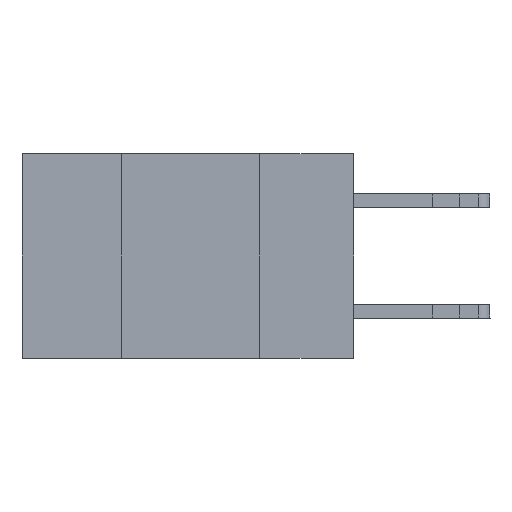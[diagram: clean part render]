
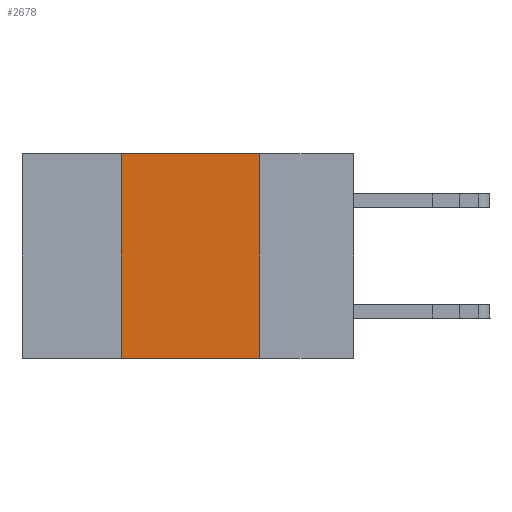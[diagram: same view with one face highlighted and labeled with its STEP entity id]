
A CAD part, left-side view. The second image highlights one B-rep face of the part: STEP entity #2678.
In plain terms, the highlighted planar face has unit normal (-1, 0, 0).
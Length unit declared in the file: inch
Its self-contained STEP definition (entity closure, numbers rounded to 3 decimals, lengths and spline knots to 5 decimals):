
#125 = CARTESIAN_POINT ( 'NONE',  ( 0., 0.6, -0.37 ) ) ;
#500 = FACE_OUTER_BOUND ( 'NONE', #3362, .T. ) ;
#575 = PLANE ( 'NONE',  #9964 ) ;
#965 = LINE ( 'NONE', #12257, #12433 ) ;
#1796 = ORIENTED_EDGE ( 'NONE', *, *, #3652, .F. ) ;
#2283 = VECTOR ( 'NONE', #12940, 39.37008 ) ;
#2678 = ADVANCED_FACE ( 'NONE', ( #500 ), #575, .F. ) ;
#3362 = EDGE_LOOP ( 'NONE', ( #1796, #6665, #6150, #10160 ) ) ;
#3477 = CARTESIAN_POINT ( 'NONE',  ( 0., 0.42, -0.37 ) ) ;
#3588 = VECTOR ( 'NONE', #4647, 39.37008 ) ;
#3652 = EDGE_CURVE ( 'NONE', #11167, #9897, #965, .T. ) ;
#4084 = CARTESIAN_POINT ( 'NONE',  ( 0., 0.17, -0.37 ) ) ;
#4290 = DIRECTION ( 'NONE',  ( 0., 0., -1. ) ) ;
#4377 = CARTESIAN_POINT ( 'NONE',  ( 0., 0.42, 0. ) ) ;
#4647 = DIRECTION ( 'NONE',  ( 0., -1., 0. ) ) ;
#5505 = VERTEX_POINT ( 'NONE', #3477 ) ;
#5913 = CARTESIAN_POINT ( 'NONE',  ( 0., 0.17, 0. ) ) ;
#6150 = ORIENTED_EDGE ( 'NONE', *, *, #13628, .F. ) ;
#6251 = VECTOR ( 'NONE', #9463, 39.37008 ) ;
#6665 = ORIENTED_EDGE ( 'NONE', *, *, #8636, .F. ) ;
#8440 = VERTEX_POINT ( 'NONE', #14270 ) ;
#8636 = EDGE_CURVE ( 'NONE', #8440, #11167, #16098, .T. ) ;
#8903 = LINE ( 'NONE', #125, #2283 ) ;
#9463 = DIRECTION ( 'NONE',  ( 0., 0., 1. ) ) ;
#9625 = LINE ( 'NONE', #4377, #6251 ) ;
#9731 = DIRECTION ( 'NONE',  ( 0., 0., -1. ) ) ;
#9897 = VERTEX_POINT ( 'NONE', #4084 ) ;
#9964 = AXIS2_PLACEMENT_3D ( 'NONE', #10852, #15750, #4290 ) ;
#10160 = ORIENTED_EDGE ( 'NONE', *, *, #14320, .T. ) ;
#10852 = CARTESIAN_POINT ( 'NONE',  ( 0., 0.6, 0. ) ) ;
#11167 = VERTEX_POINT ( 'NONE', #5913 ) ;
#12257 = CARTESIAN_POINT ( 'NONE',  ( 0., 0.17, 0. ) ) ;
#12433 = VECTOR ( 'NONE', #9731, 39.37008 ) ;
#12940 = DIRECTION ( 'NONE',  ( 0., -1., 0. ) ) ;
#13628 = EDGE_CURVE ( 'NONE', #5505, #8440, #9625, .T. ) ;
#14270 = CARTESIAN_POINT ( 'NONE',  ( 0., 0.42, 0. ) ) ;
#14320 = EDGE_CURVE ( 'NONE', #5505, #9897, #8903, .T. ) ;
#14856 = CARTESIAN_POINT ( 'NONE',  ( 0., 0.6, 0. ) ) ;
#15750 = DIRECTION ( 'NONE',  ( 1., 0., 0. ) ) ;
#16098 = LINE ( 'NONE', #14856, #3588 ) ;
